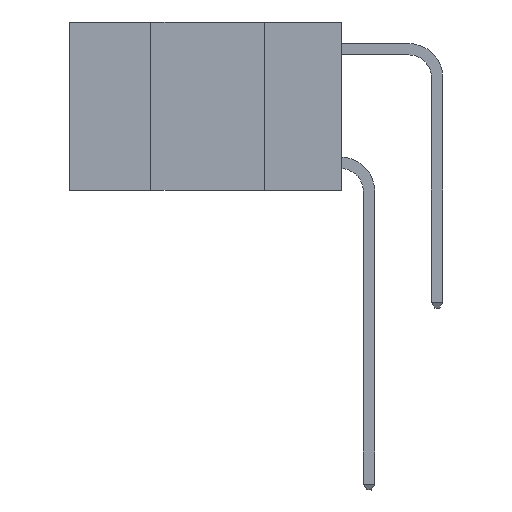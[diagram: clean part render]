
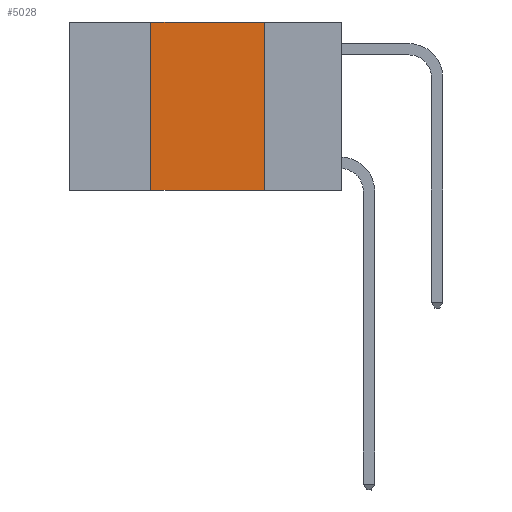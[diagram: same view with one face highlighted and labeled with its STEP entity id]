
A CAD part, left-side view. The second image highlights one B-rep face of the part: STEP entity #5028.
In plain terms, the highlighted planar face has unit normal (-1, 0, 0).
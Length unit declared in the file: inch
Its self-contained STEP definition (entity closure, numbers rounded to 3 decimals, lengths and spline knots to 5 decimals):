
#460 = EDGE_CURVE ( 'NONE', #2532, #2850, #14662, .T. ) ;
#1619 = LINE ( 'NONE', #3769, #18182 ) ;
#1709 = VECTOR ( 'NONE', #13561, 39.37008 ) ;
#2532 = VERTEX_POINT ( 'NONE', #4031 ) ;
#2631 = CARTESIAN_POINT ( 'NONE',  ( 0., 0.6, -0.37 ) ) ;
#2678 = LINE ( 'NONE', #6781, #10848 ) ;
#2850 = VERTEX_POINT ( 'NONE', #17561 ) ;
#3769 = CARTESIAN_POINT ( 'NONE',  ( 0., 0.42, 0. ) ) ;
#4031 = CARTESIAN_POINT ( 'NONE',  ( 0., 0.42, 0. ) ) ;
#5028 = ADVANCED_FACE ( 'NONE', ( #17389 ), #7041, .F. ) ;
#5423 = DIRECTION ( 'NONE',  ( 1., 0., 0. ) ) ;
#6781 = CARTESIAN_POINT ( 'NONE',  ( 0., 0.17, 0. ) ) ;
#7041 = PLANE ( 'NONE',  #9233 ) ;
#7051 = CARTESIAN_POINT ( 'NONE',  ( 0., 0.6, 0. ) ) ;
#8417 = DIRECTION ( 'NONE',  ( 0., 0., -1. ) ) ;
#8524 = EDGE_LOOP ( 'NONE', ( #9752, #9874, #9920, #10298 ) ) ;
#8650 = DIRECTION ( 'NONE',  ( 0., 0., 1. ) ) ;
#9233 = AXIS2_PLACEMENT_3D ( 'NONE', #11923, #5423, #16653 ) ;
#9752 = ORIENTED_EDGE ( 'NONE', *, *, #19726, .F. ) ;
#9874 = ORIENTED_EDGE ( 'NONE', *, *, #460, .F. ) ;
#9920 = ORIENTED_EDGE ( 'NONE', *, *, #14602, .F. ) ;
#10180 = VERTEX_POINT ( 'NONE', #16427 ) ;
#10298 = ORIENTED_EDGE ( 'NONE', *, *, #12478, .T. ) ;
#10490 = CARTESIAN_POINT ( 'NONE',  ( 0., 0.17, -0.37 ) ) ;
#10848 = VECTOR ( 'NONE', #8417, 39.37008 ) ;
#11923 = CARTESIAN_POINT ( 'NONE',  ( 0., 0.6, 0. ) ) ;
#12478 = EDGE_CURVE ( 'NONE', #10180, #16490, #18368, .T. ) ;
#13561 = DIRECTION ( 'NONE',  ( 0., -1., 0. ) ) ;
#14077 = DIRECTION ( 'NONE',  ( 0., -1., 0. ) ) ;
#14271 = VECTOR ( 'NONE', #14077, 39.37008 ) ;
#14602 = EDGE_CURVE ( 'NONE', #10180, #2532, #1619, .T. ) ;
#14662 = LINE ( 'NONE', #7051, #1709 ) ;
#16427 = CARTESIAN_POINT ( 'NONE',  ( 0., 0.42, -0.37 ) ) ;
#16490 = VERTEX_POINT ( 'NONE', #10490 ) ;
#16653 = DIRECTION ( 'NONE',  ( 0., 0., -1. ) ) ;
#17389 = FACE_OUTER_BOUND ( 'NONE', #8524, .T. ) ;
#17561 = CARTESIAN_POINT ( 'NONE',  ( 0., 0.17, 0. ) ) ;
#18182 = VECTOR ( 'NONE', #8650, 39.37008 ) ;
#18368 = LINE ( 'NONE', #2631, #14271 ) ;
#19726 = EDGE_CURVE ( 'NONE', #2850, #16490, #2678, .T. ) ;
